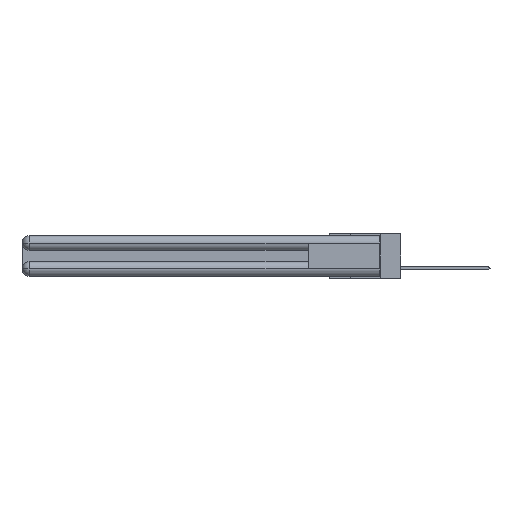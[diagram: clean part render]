
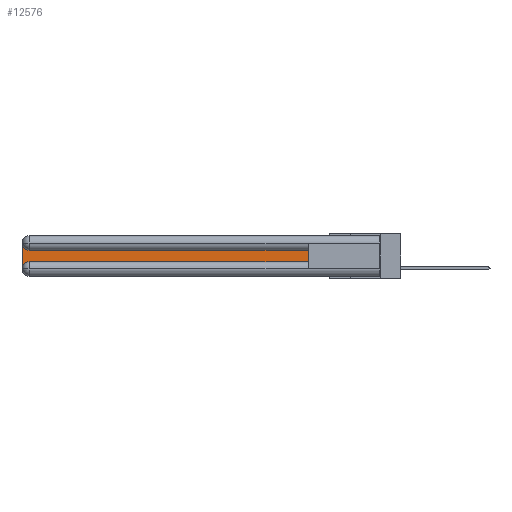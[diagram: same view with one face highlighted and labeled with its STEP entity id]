
A CAD part, left-side view. The second image highlights one B-rep face of the part: STEP entity #12576.
In plain terms, the highlighted planar face has unit normal (-1, 0, 0).
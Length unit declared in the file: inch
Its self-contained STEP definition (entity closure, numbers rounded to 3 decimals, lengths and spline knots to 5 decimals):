
#970 = VECTOR ( 'NONE', #32354, 39.37008 ) ;
#1292 = CARTESIAN_POINT ( 'NONE',  ( 0.075, 2.94, -0.2175 ) ) ;
#1377 = DIRECTION ( 'NONE',  ( 0., 0., -1. ) ) ;
#1866 = ORIENTED_EDGE ( 'NONE', *, *, #7931, .T. ) ;
#4877 = CARTESIAN_POINT ( 'NONE',  ( 0.075, 3., -0.2175 ) ) ;
#4878 = AXIS2_PLACEMENT_3D ( 'NONE', #11660, #6104, #1377 ) ;
#5515 = LINE ( 'NONE', #15806, #32136 ) ;
#6104 = DIRECTION ( 'NONE',  ( 1., 0., 0. ) ) ;
#7163 = DIRECTION ( 'NONE',  ( 0., 0., -1. ) ) ;
#7931 = EDGE_CURVE ( 'NONE', #22534, #15778, #17602, .T. ) ;
#8270 = LINE ( 'NONE', #19054, #970 ) ;
#8368 = VERTEX_POINT ( 'NONE', #28304 ) ;
#8524 = EDGE_CURVE ( 'NONE', #30836, #21559, #8270, .T. ) ;
#9873 = DIRECTION ( 'NONE',  ( 0., 0., 1. ) ) ;
#10220 = ORIENTED_EDGE ( 'NONE', *, *, #31986, .T. ) ;
#10236 = CIRCLE ( 'NONE', #30492, 0.06 ) ;
#11660 = CARTESIAN_POINT ( 'NONE',  ( 0.075, 3., -0.1225 ) ) ;
#12576 = ADVANCED_FACE ( 'NONE', ( #26727 ), #24448, .F. ) ;
#14189 = VERTEX_POINT ( 'NONE', #1292 ) ;
#15778 = VERTEX_POINT ( 'NONE', #20936 ) ;
#15806 = CARTESIAN_POINT ( 'NONE',  ( 0.075, 0.6, -0.2175 ) ) ;
#16049 = DIRECTION ( 'NONE',  ( 1., 0., 0. ) ) ;
#16948 = LINE ( 'NONE', #17445, #29813 ) ;
#17445 = CARTESIAN_POINT ( 'NONE',  ( 0.075, 0.6, -0.2175 ) ) ;
#17463 = EDGE_CURVE ( 'NONE', #21559, #22534, #21633, .T. ) ;
#17602 = LINE ( 'NONE', #4877, #20779 ) ;
#17923 = ORIENTED_EDGE ( 'NONE', *, *, #27471, .T. ) ;
#18276 = DIRECTION ( 'NONE',  ( 0., 0., -1. ) ) ;
#18347 = AXIS2_PLACEMENT_3D ( 'NONE', #28752, #16049, #18595 ) ;
#18595 = DIRECTION ( 'NONE',  ( 0., 0., -1. ) ) ;
#19054 = CARTESIAN_POINT ( 'NONE',  ( 0.075, 0.6, -0.1225 ) ) ;
#19132 = CARTESIAN_POINT ( 'NONE',  ( 0.075, 0.6, -0.1225 ) ) ;
#20779 = VECTOR ( 'NONE', #18276, 39.37008 ) ;
#20936 = CARTESIAN_POINT ( 'NONE',  ( 0.075, 3., -0.2775 ) ) ;
#21559 = VERTEX_POINT ( 'NONE', #27620 ) ;
#21633 = CIRCLE ( 'NONE', #18347, 0.06 ) ;
#22534 = VERTEX_POINT ( 'NONE', #29109 ) ;
#23092 = DIRECTION ( 'NONE',  ( 0., -1., 0. ) ) ;
#23251 = ORIENTED_EDGE ( 'NONE', *, *, #17463, .T. ) ;
#24448 = PLANE ( 'NONE',  #4878 ) ;
#24944 = EDGE_LOOP ( 'NONE', ( #32350, #23251, #1866, #10220, #26744, #17923 ) ) ;
#24949 = DIRECTION ( 'NONE',  ( 1., 0., 0. ) ) ;
#26727 = FACE_OUTER_BOUND ( 'NONE', #24944, .T. ) ;
#26744 = ORIENTED_EDGE ( 'NONE', *, *, #29986, .T. ) ;
#27471 = EDGE_CURVE ( 'NONE', #8368, #30836, #16948, .T. ) ;
#27620 = CARTESIAN_POINT ( 'NONE',  ( 0.075, 2.94, -0.1225 ) ) ;
#28304 = CARTESIAN_POINT ( 'NONE',  ( 0.075, 0.6, -0.2175 ) ) ;
#28752 = CARTESIAN_POINT ( 'NONE',  ( 0.075, 2.94, -0.0625 ) ) ;
#29109 = CARTESIAN_POINT ( 'NONE',  ( 0.075, 3., -0.0625 ) ) ;
#29813 = VECTOR ( 'NONE', #9873, 39.37008 ) ;
#29986 = EDGE_CURVE ( 'NONE', #14189, #8368, #5515, .T. ) ;
#30492 = AXIS2_PLACEMENT_3D ( 'NONE', #32663, #24949, #7163 ) ;
#30836 = VERTEX_POINT ( 'NONE', #19132 ) ;
#31986 = EDGE_CURVE ( 'NONE', #15778, #14189, #10236, .T. ) ;
#32136 = VECTOR ( 'NONE', #23092, 39.37008 ) ;
#32350 = ORIENTED_EDGE ( 'NONE', *, *, #8524, .T. ) ;
#32354 = DIRECTION ( 'NONE',  ( 0., 1., 0. ) ) ;
#32663 = CARTESIAN_POINT ( 'NONE',  ( 0.075, 2.94, -0.2775 ) ) ;
